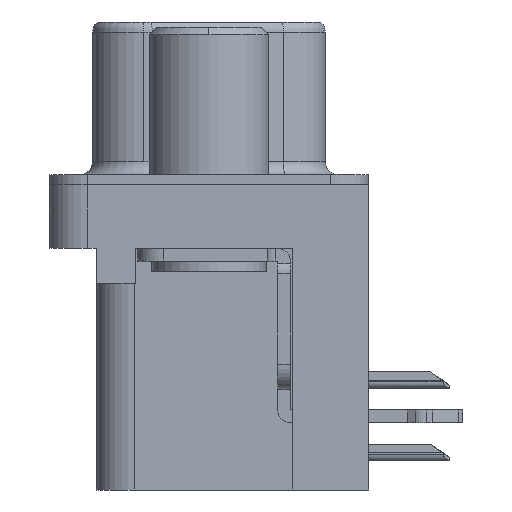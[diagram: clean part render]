
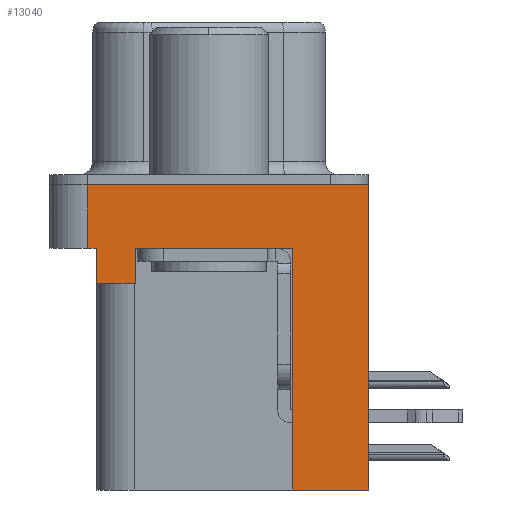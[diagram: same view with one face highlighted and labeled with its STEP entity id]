
A CAD part, left-side view. The second image highlights one B-rep face of the part: STEP entity #13040.
In plain terms, the highlighted planar face has unit normal (-1, 0, 0).
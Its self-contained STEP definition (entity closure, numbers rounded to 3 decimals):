
#822 = ORIENTED_EDGE ( 'NONE', *, *, #7501, .T. ) ;
#1000 = EDGE_LOOP ( 'NONE', ( #10571, #17967, #9627, #8534, #5469, #16918, #19729, #12207, #2862, #822 ) ) ;
#1071 = CARTESIAN_POINT ( 'NONE',  ( -3., -6.275, -12. ) ) ;
#1577 = LINE ( 'NONE', #17242, #11723 ) ;
#2026 = VECTOR ( 'NONE', #8018, 1000. ) ;
#2229 = VERTEX_POINT ( 'NONE', #13439 ) ;
#2359 = DIRECTION ( 'NONE',  ( 0., 0., 1. ) ) ;
#2862 = ORIENTED_EDGE ( 'NONE', *, *, #13025, .F. ) ;
#2874 = CARTESIAN_POINT ( 'NONE',  ( -3., -3.295, -12. ) ) ;
#2895 = EDGE_CURVE ( 'NONE', #18621, #18198, #19145, .T. ) ;
#3177 = CARTESIAN_POINT ( 'NONE',  ( -3., 4.425, -3.9 ) ) ;
#3848 = FACE_OUTER_BOUND ( 'NONE', #1000, .T. ) ;
#4334 = CARTESIAN_POINT ( 'NONE',  ( -3., -6.275, -2.5 ) ) ;
#4682 = EDGE_CURVE ( 'NONE', #7104, #2229, #13115, .T. ) ;
#4803 = PLANE ( 'NONE',  #16913 ) ;
#5121 = CARTESIAN_POINT ( 'NONE',  ( -3., -6.275, -2.5 ) ) ;
#5134 = VECTOR ( 'NONE', #17184, 1000. ) ;
#5139 = LINE ( 'NONE', #5121, #18441 ) ;
#5469 = ORIENTED_EDGE ( 'NONE', *, *, #23329, .F. ) ;
#5644 = DIRECTION ( 'NONE',  ( 0., 0., 1. ) ) ;
#6079 = CARTESIAN_POINT ( 'NONE',  ( -3., -6.275, -2.5 ) ) ;
#6115 = DIRECTION ( 'NONE',  ( 0., -1., 0. ) ) ;
#6537 = DIRECTION ( 'NONE',  ( -1., 0., 0. ) ) ;
#7104 = VERTEX_POINT ( 'NONE', #15354 ) ;
#7197 = CARTESIAN_POINT ( 'NONE',  ( -3., 4.425, -2.5 ) ) ;
#7413 = CARTESIAN_POINT ( 'NONE',  ( -3., 4.775, 0. ) ) ;
#7501 = EDGE_CURVE ( 'NONE', #7758, #10305, #12176, .T. ) ;
#7758 = VERTEX_POINT ( 'NONE', #1071 ) ;
#7895 = CARTESIAN_POINT ( 'NONE',  ( -3., -6.275, 0. ) ) ;
#8018 = DIRECTION ( 'NONE',  ( 0., 0., 1. ) ) ;
#8304 = VECTOR ( 'NONE', #10086, 1000. ) ;
#8534 = ORIENTED_EDGE ( 'NONE', *, *, #17347, .F. ) ;
#8808 = DIRECTION ( 'NONE',  ( 0., -1., 0. ) ) ;
#9087 = CARTESIAN_POINT ( 'NONE',  ( -3., -3.295, -2.5 ) ) ;
#9627 = ORIENTED_EDGE ( 'NONE', *, *, #21103, .T. ) ;
#9904 = CARTESIAN_POINT ( 'NONE',  ( -3., -6.275, -2.5 ) ) ;
#10086 = DIRECTION ( 'NONE',  ( 0., 0., 1. ) ) ;
#10305 = VERTEX_POINT ( 'NONE', #13191 ) ;
#10571 = ORIENTED_EDGE ( 'NONE', *, *, #15043, .F. ) ;
#11723 = VECTOR ( 'NONE', #22783, 1000. ) ;
#11729 = LINE ( 'NONE', #12802, #14271 ) ;
#12176 = LINE ( 'NONE', #6079, #2026 ) ;
#12207 = ORIENTED_EDGE ( 'NONE', *, *, #12440, .F. ) ;
#12440 = EDGE_CURVE ( 'NONE', #23384, #16692, #18008, .T. ) ;
#12802 = CARTESIAN_POINT ( 'NONE',  ( -3., 4.425, -3.9 ) ) ;
#13025 = EDGE_CURVE ( 'NONE', #7758, #23384, #1577, .T. ) ;
#13040 = ADVANCED_FACE ( 'NONE', ( #3848 ), #4803, .T. ) ;
#13115 = LINE ( 'NONE', #17412, #8304 ) ;
#13191 = CARTESIAN_POINT ( 'NONE',  ( -3., -6.275, 0. ) ) ;
#13439 = CARTESIAN_POINT ( 'NONE',  ( -3., 2.895, -2.5 ) ) ;
#14271 = VECTOR ( 'NONE', #2359, 1000. ) ;
#14371 = LINE ( 'NONE', #4334, #21144 ) ;
#15043 = EDGE_CURVE ( 'NONE', #18198, #10305, #21244, .T. ) ;
#15354 = CARTESIAN_POINT ( 'NONE',  ( -3., 2.895, -3.9 ) ) ;
#16692 = VERTEX_POINT ( 'NONE', #9087 ) ;
#16744 = LINE ( 'NONE', #18819, #5134 ) ;
#16913 = AXIS2_PLACEMENT_3D ( 'NONE', #9904, #6537, #19015 ) ;
#16918 = ORIENTED_EDGE ( 'NONE', *, *, #4682, .T. ) ;
#17184 = DIRECTION ( 'NONE',  ( 0., 1., 0. ) ) ;
#17242 = CARTESIAN_POINT ( 'NONE',  ( -3., -3.295, -12. ) ) ;
#17347 = EDGE_CURVE ( 'NONE', #20884, #17622, #11729, .T. ) ;
#17349 = CARTESIAN_POINT ( 'NONE',  ( -3., -3.295, -12. ) ) ;
#17412 = CARTESIAN_POINT ( 'NONE',  ( -3., 2.895, -3.9 ) ) ;
#17622 = VERTEX_POINT ( 'NONE', #7197 ) ;
#17967 = ORIENTED_EDGE ( 'NONE', *, *, #2895, .F. ) ;
#18008 = LINE ( 'NONE', #17349, #18827 ) ;
#18198 = VERTEX_POINT ( 'NONE', #7413 ) ;
#18441 = VECTOR ( 'NONE', #8808, 1000. ) ;
#18453 = VECTOR ( 'NONE', #6115, 1000. ) ;
#18621 = VERTEX_POINT ( 'NONE', #23136 ) ;
#18819 = CARTESIAN_POINT ( 'NONE',  ( -3., 4.425, -3.9 ) ) ;
#18827 = VECTOR ( 'NONE', #21300, 1000. ) ;
#18866 = DIRECTION ( 'NONE',  ( 0., -1., 0. ) ) ;
#19015 = DIRECTION ( 'NONE',  ( 0., 0., 1. ) ) ;
#19145 = LINE ( 'NONE', #21893, #19965 ) ;
#19420 = EDGE_CURVE ( 'NONE', #2229, #16692, #5139, .T. ) ;
#19729 = ORIENTED_EDGE ( 'NONE', *, *, #19420, .T. ) ;
#19965 = VECTOR ( 'NONE', #5644, 1000. ) ;
#20884 = VERTEX_POINT ( 'NONE', #3177 ) ;
#21103 = EDGE_CURVE ( 'NONE', #18621, #17622, #14371, .T. ) ;
#21144 = VECTOR ( 'NONE', #18866, 1000. ) ;
#21244 = LINE ( 'NONE', #7895, #18453 ) ;
#21300 = DIRECTION ( 'NONE',  ( 0., 0., 1. ) ) ;
#21893 = CARTESIAN_POINT ( 'NONE',  ( -3., 4.775, -2.5 ) ) ;
#22783 = DIRECTION ( 'NONE',  ( 0., 1., 0. ) ) ;
#23136 = CARTESIAN_POINT ( 'NONE',  ( -3., 4.775, -2.5 ) ) ;
#23329 = EDGE_CURVE ( 'NONE', #7104, #20884, #16744, .T. ) ;
#23384 = VERTEX_POINT ( 'NONE', #2874 ) ;
